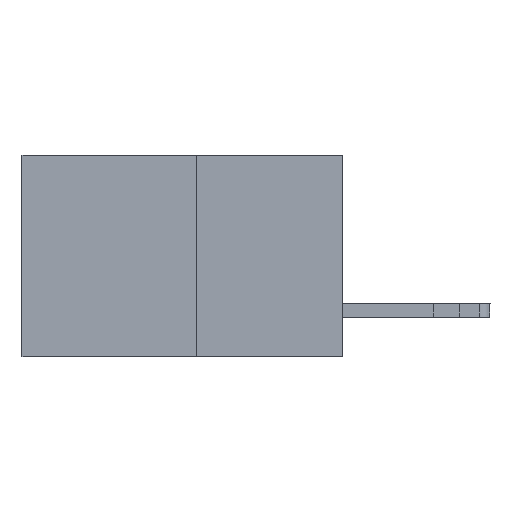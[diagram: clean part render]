
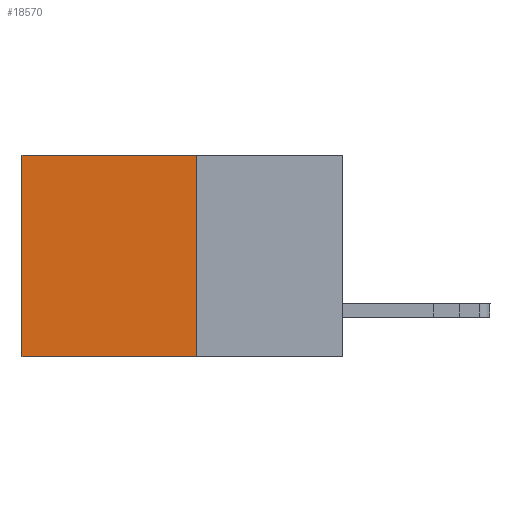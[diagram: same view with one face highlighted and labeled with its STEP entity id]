
A CAD part, left-side view. The second image highlights one B-rep face of the part: STEP entity #18570.
In plain terms, the highlighted planar face has unit normal (-1, 0, 0).
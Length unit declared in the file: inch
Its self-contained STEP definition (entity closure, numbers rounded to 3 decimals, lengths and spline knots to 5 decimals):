
#169 = ORIENTED_EDGE ( 'NONE', *, *, #20807, .T. ) ;
#192 = CARTESIAN_POINT ( 'NONE',  ( 0.277, 0.27, -0.37 ) ) ;
#844 = ORIENTED_EDGE ( 'NONE', *, *, #6161, .F. ) ;
#2507 = CARTESIAN_POINT ( 'NONE',  ( 0.277, 0.27, -0.37 ) ) ;
#3072 = DIRECTION ( 'NONE',  ( 0., 0., -1. ) ) ;
#3472 = VECTOR ( 'NONE', #16008, 39.37008 ) ;
#4957 = VERTEX_POINT ( 'NONE', #192 ) ;
#5341 = DIRECTION ( 'NONE',  ( 0., 0., -1. ) ) ;
#6161 = EDGE_CURVE ( 'NONE', #4957, #23150, #18490, .T. ) ;
#6260 = CARTESIAN_POINT ( 'NONE',  ( 0.277, 0.27, 0. ) ) ;
#7457 = PLANE ( 'NONE',  #30776 ) ;
#8119 = VECTOR ( 'NONE', #3072, 39.37008 ) ;
#9164 = CARTESIAN_POINT ( 'NONE',  ( 0.277, 0.59, 0. ) ) ;
#9288 = LINE ( 'NONE', #6260, #3472 ) ;
#9411 = CARTESIAN_POINT ( 'NONE',  ( 0.277, 0.27, -0.37 ) ) ;
#10224 = CARTESIAN_POINT ( 'NONE',  ( 0.277, 0.27, -0.37 ) ) ;
#11909 = ORIENTED_EDGE ( 'NONE', *, *, #20619, .T. ) ;
#12066 = VECTOR ( 'NONE', #14699, 39.37008 ) ;
#12217 = ORIENTED_EDGE ( 'NONE', *, *, #16390, .F. ) ;
#12391 = DIRECTION ( 'NONE',  ( 0., 0., -1. ) ) ;
#14253 = VECTOR ( 'NONE', #5341, 39.37008 ) ;
#14699 = DIRECTION ( 'NONE',  ( 0., 1., 0. ) ) ;
#15060 = CARTESIAN_POINT ( 'NONE',  ( 0.277, 0.27, 0. ) ) ;
#16008 = DIRECTION ( 'NONE',  ( 0., 1., 0. ) ) ;
#16390 = EDGE_CURVE ( 'NONE', #20555, #4957, #27061, .T. ) ;
#17692 = VERTEX_POINT ( 'NONE', #9164 ) ;
#18490 = LINE ( 'NONE', #9411, #12066 ) ;
#18570 = ADVANCED_FACE ( 'NONE', ( #18881 ), #7457, .F. ) ;
#18881 = FACE_OUTER_BOUND ( 'NONE', #29163, .T. ) ;
#20110 = CARTESIAN_POINT ( 'NONE',  ( 0.277, 0.59, -0.37 ) ) ;
#20555 = VERTEX_POINT ( 'NONE', #15060 ) ;
#20619 = EDGE_CURVE ( 'NONE', #17692, #23150, #27420, .T. ) ;
#20807 = EDGE_CURVE ( 'NONE', #20555, #17692, #9288, .T. ) ;
#23150 = VERTEX_POINT ( 'NONE', #24213 ) ;
#24213 = CARTESIAN_POINT ( 'NONE',  ( 0.277, 0.59, -0.37 ) ) ;
#26834 = DIRECTION ( 'NONE',  ( 1., 0., 0. ) ) ;
#27061 = LINE ( 'NONE', #10224, #14253 ) ;
#27420 = LINE ( 'NONE', #20110, #8119 ) ;
#29163 = EDGE_LOOP ( 'NONE', ( #11909, #844, #12217, #169 ) ) ;
#30776 = AXIS2_PLACEMENT_3D ( 'NONE', #2507, #26834, #12391 ) ;
